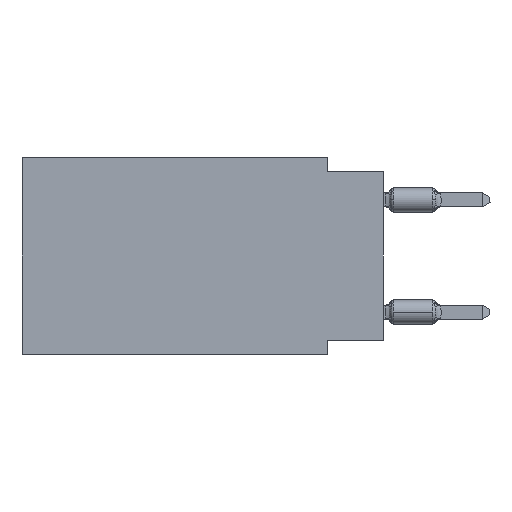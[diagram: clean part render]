
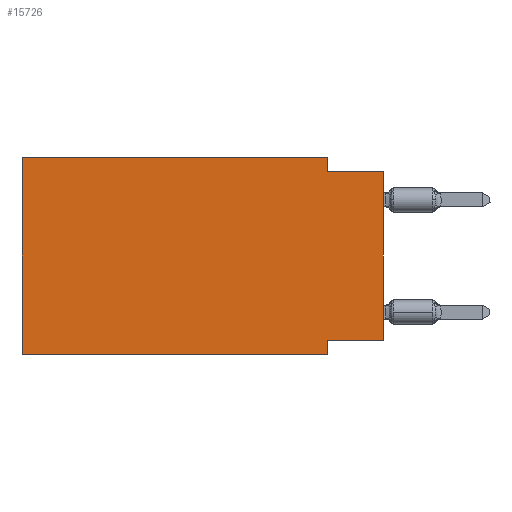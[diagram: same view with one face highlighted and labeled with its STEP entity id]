
A CAD part, left-side view. The second image highlights one B-rep face of the part: STEP entity #15726.
In plain terms, the highlighted planar face has unit normal (-1, 0, 0).
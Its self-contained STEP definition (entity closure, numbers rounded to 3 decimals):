
#805 = DIRECTION ( 'NONE',  ( 0., 0., -1. ) ) ;
#1982 = CARTESIAN_POINT ( 'NONE',  ( 0., 0., 0. ) ) ;
#2332 = DIRECTION ( 'NONE',  ( 1., 0., 0. ) ) ;
#2355 = VECTOR ( 'NONE', #27024, 1000. ) ;
#4946 = CARTESIAN_POINT ( 'NONE',  ( 0., 2.54, 0. ) ) ;
#5226 = EDGE_CURVE ( 'NONE', #25252, #28619, #23733, .T. ) ;
#5980 = ORIENTED_EDGE ( 'NONE', *, *, #22745, .T. ) ;
#7901 = AXIS2_PLACEMENT_3D ( 'NONE', #17694, #2332, #20734 ) ;
#8541 = CARTESIAN_POINT ( 'NONE',  ( 0., 0., -0.635 ) ) ;
#8858 = DIRECTION ( 'NONE',  ( 0., -1., 0. ) ) ;
#9612 = VERTEX_POINT ( 'NONE', #12018 ) ;
#10079 = CARTESIAN_POINT ( 'NONE',  ( 0., 2.54, -8.255 ) ) ;
#10483 = EDGE_CURVE ( 'NONE', #23478, #25252, #21375, .T. ) ;
#10760 = DIRECTION ( 'NONE',  ( 0., 0., 1. ) ) ;
#11537 = DIRECTION ( 'NONE',  ( 0., -1., 0. ) ) ;
#12018 = CARTESIAN_POINT ( 'NONE',  ( 0., 16.383, -8.89 ) ) ;
#12754 = DIRECTION ( 'NONE',  ( 0., 1., 0. ) ) ;
#14354 = EDGE_CURVE ( 'NONE', #26264, #33459, #16757, .T. ) ;
#14753 = ORIENTED_EDGE ( 'NONE', *, *, #22020, .F. ) ;
#15611 = LINE ( 'NONE', #30068, #2355 ) ;
#15726 = ADVANCED_FACE ( 'NONE', ( #25176 ), #16622, .F. ) ;
#15779 = VECTOR ( 'NONE', #12754, 1000. ) ;
#15950 = ORIENTED_EDGE ( 'NONE', *, *, #30539, .T. ) ;
#16560 = ORIENTED_EDGE ( 'NONE', *, *, #5226, .F. ) ;
#16622 = PLANE ( 'NONE',  #7901 ) ;
#16757 = LINE ( 'NONE', #22283, #29151 ) ;
#17201 = VECTOR ( 'NONE', #34957, 1000. ) ;
#17292 = CARTESIAN_POINT ( 'NONE',  ( 0., 2.54, -8.89 ) ) ;
#17694 = CARTESIAN_POINT ( 'NONE',  ( 0., 16.383, 0. ) ) ;
#19131 = EDGE_CURVE ( 'NONE', #27168, #23478, #23301, .T. ) ;
#19605 = ORIENTED_EDGE ( 'NONE', *, *, #19131, .F. ) ;
#19610 = DIRECTION ( 'NONE',  ( 0., 0., -1. ) ) ;
#19711 = VECTOR ( 'NONE', #805, 1000. ) ;
#20107 = ORIENTED_EDGE ( 'NONE', *, *, #10483, .F. ) ;
#20734 = DIRECTION ( 'NONE',  ( 0., 0., -1. ) ) ;
#21315 = LINE ( 'NONE', #32905, #15779 ) ;
#21375 = LINE ( 'NONE', #30513, #19711 ) ;
#22020 = EDGE_CURVE ( 'NONE', #9612, #27168, #15611, .T. ) ;
#22206 = VECTOR ( 'NONE', #11537, 1000. ) ;
#22283 = CARTESIAN_POINT ( 'NONE',  ( 0., 2.54, -8.89 ) ) ;
#22557 = ORIENTED_EDGE ( 'NONE', *, *, #29512, .F. ) ;
#22745 = EDGE_CURVE ( 'NONE', #9612, #33459, #34012, .T. ) ;
#23301 = LINE ( 'NONE', #26728, #30881 ) ;
#23478 = VERTEX_POINT ( 'NONE', #4946 ) ;
#23733 = LINE ( 'NONE', #29258, #17201 ) ;
#25176 = FACE_OUTER_BOUND ( 'NONE', #27073, .T. ) ;
#25252 = VERTEX_POINT ( 'NONE', #25290 ) ;
#25290 = CARTESIAN_POINT ( 'NONE',  ( 0., 2.54, -0.635 ) ) ;
#26264 = VERTEX_POINT ( 'NONE', #10079 ) ;
#26654 = VERTEX_POINT ( 'NONE', #30588 ) ;
#26728 = CARTESIAN_POINT ( 'NONE',  ( 0., 16.383, 0. ) ) ;
#27024 = DIRECTION ( 'NONE',  ( 0., 0., 1. ) ) ;
#27073 = EDGE_LOOP ( 'NONE', ( #15950, #16560, #20107, #19605, #14753, #5980, #35443, #22557 ) ) ;
#27168 = VERTEX_POINT ( 'NONE', #28436 ) ;
#28117 = CARTESIAN_POINT ( 'NONE',  ( 0., 16.383, -8.89 ) ) ;
#28436 = CARTESIAN_POINT ( 'NONE',  ( 0., 16.383, 0. ) ) ;
#28619 = VERTEX_POINT ( 'NONE', #8541 ) ;
#29151 = VECTOR ( 'NONE', #19610, 1000. ) ;
#29258 = CARTESIAN_POINT ( 'NONE',  ( 0., 0., -0.635 ) ) ;
#29512 = EDGE_CURVE ( 'NONE', #26654, #26264, #21315, .T. ) ;
#30068 = CARTESIAN_POINT ( 'NONE',  ( 0., 16.383, 0. ) ) ;
#30513 = CARTESIAN_POINT ( 'NONE',  ( 0., 2.54, 0. ) ) ;
#30539 = EDGE_CURVE ( 'NONE', #26654, #28619, #36261, .T. ) ;
#30588 = CARTESIAN_POINT ( 'NONE',  ( 0., 0., -8.255 ) ) ;
#30881 = VECTOR ( 'NONE', #8858, 1000. ) ;
#32905 = CARTESIAN_POINT ( 'NONE',  ( 0., 0., -8.255 ) ) ;
#33459 = VERTEX_POINT ( 'NONE', #17292 ) ;
#34012 = LINE ( 'NONE', #28117, #22206 ) ;
#34957 = DIRECTION ( 'NONE',  ( 0., -1., 0. ) ) ;
#35443 = ORIENTED_EDGE ( 'NONE', *, *, #14354, .F. ) ;
#36261 = LINE ( 'NONE', #1982, #37103 ) ;
#37103 = VECTOR ( 'NONE', #10760, 1000. ) ;
